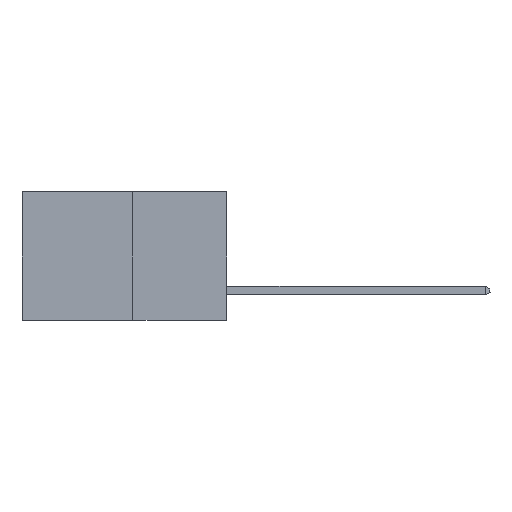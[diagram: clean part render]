
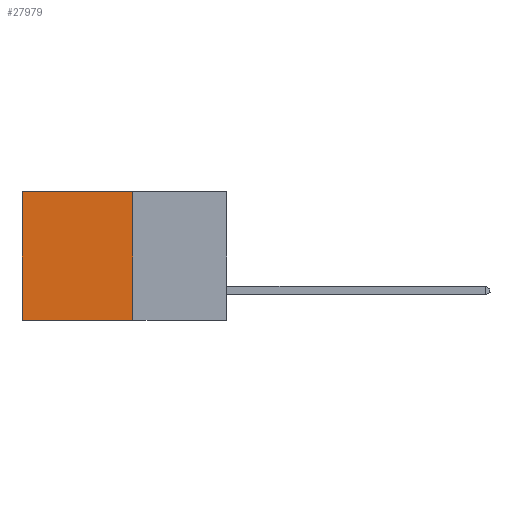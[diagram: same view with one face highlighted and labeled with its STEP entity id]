
A CAD part, left-side view. The second image highlights one B-rep face of the part: STEP entity #27979.
In plain terms, the highlighted planar face has unit normal (-1, 0, 0).
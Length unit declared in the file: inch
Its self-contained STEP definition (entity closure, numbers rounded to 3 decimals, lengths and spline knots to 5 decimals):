
#25 = EDGE_CURVE ( 'NONE', #15149, #19404, #342, .T. ) ;
#342 = LINE ( 'NONE', #5427, #23778 ) ;
#1555 = CARTESIAN_POINT ( 'NONE',  ( 0.277, 0.59, -0.37 ) ) ;
#2508 = ORIENTED_EDGE ( 'NONE', *, *, #25, .F. ) ;
#3006 = DIRECTION ( 'NONE',  ( 0., 0., -1. ) ) ;
#3864 = DIRECTION ( 'NONE',  ( 0., 0., -1. ) ) ;
#3896 = CARTESIAN_POINT ( 'NONE',  ( 0.277, 0.27, 0. ) ) ;
#4366 = VECTOR ( 'NONE', #3006, 39.37008 ) ;
#4457 = VECTOR ( 'NONE', #20375, 39.37008 ) ;
#4595 = AXIS2_PLACEMENT_3D ( 'NONE', #9220, #24940, #11522 ) ;
#4822 = LINE ( 'NONE', #1555, #10210 ) ;
#5427 = CARTESIAN_POINT ( 'NONE',  ( 0.277, 0.27, -0.37 ) ) ;
#5848 = DIRECTION ( 'NONE',  ( 0., 1., 0. ) ) ;
#5907 = LINE ( 'NONE', #24860, #4457 ) ;
#9220 = CARTESIAN_POINT ( 'NONE',  ( 0.277, 0.27, -0.37 ) ) ;
#10210 = VECTOR ( 'NONE', #3864, 39.37008 ) ;
#10757 = CARTESIAN_POINT ( 'NONE',  ( 0.277, 0.27, -0.37 ) ) ;
#10830 = FACE_OUTER_BOUND ( 'NONE', #16677, .T. ) ;
#11522 = DIRECTION ( 'NONE',  ( 0., 0., -1. ) ) ;
#11922 = CARTESIAN_POINT ( 'NONE',  ( 0.277, 0.59, 0. ) ) ;
#12975 = ORIENTED_EDGE ( 'NONE', *, *, #17536, .F. ) ;
#14118 = EDGE_CURVE ( 'NONE', #21661, #19404, #4822, .T. ) ;
#14358 = CARTESIAN_POINT ( 'NONE',  ( 0.277, 0.27, -0.37 ) ) ;
#15149 = VERTEX_POINT ( 'NONE', #10757 ) ;
#16677 = EDGE_LOOP ( 'NONE', ( #21957, #2508, #12975, #29002 ) ) ;
#16843 = CARTESIAN_POINT ( 'NONE',  ( 0.277, 0.59, -0.37 ) ) ;
#17536 = EDGE_CURVE ( 'NONE', #28364, #15149, #28312, .T. ) ;
#19404 = VERTEX_POINT ( 'NONE', #16843 ) ;
#20375 = DIRECTION ( 'NONE',  ( 0., 1., 0. ) ) ;
#21661 = VERTEX_POINT ( 'NONE', #11922 ) ;
#21957 = ORIENTED_EDGE ( 'NONE', *, *, #14118, .T. ) ;
#22711 = PLANE ( 'NONE',  #4595 ) ;
#23778 = VECTOR ( 'NONE', #5848, 39.37008 ) ;
#24860 = CARTESIAN_POINT ( 'NONE',  ( 0.277, 0.27, 0. ) ) ;
#24940 = DIRECTION ( 'NONE',  ( 1., 0., 0. ) ) ;
#26548 = EDGE_CURVE ( 'NONE', #28364, #21661, #5907, .T. ) ;
#27979 = ADVANCED_FACE ( 'NONE', ( #10830 ), #22711, .F. ) ;
#28312 = LINE ( 'NONE', #14358, #4366 ) ;
#28364 = VERTEX_POINT ( 'NONE', #3896 ) ;
#29002 = ORIENTED_EDGE ( 'NONE', *, *, #26548, .T. ) ;
